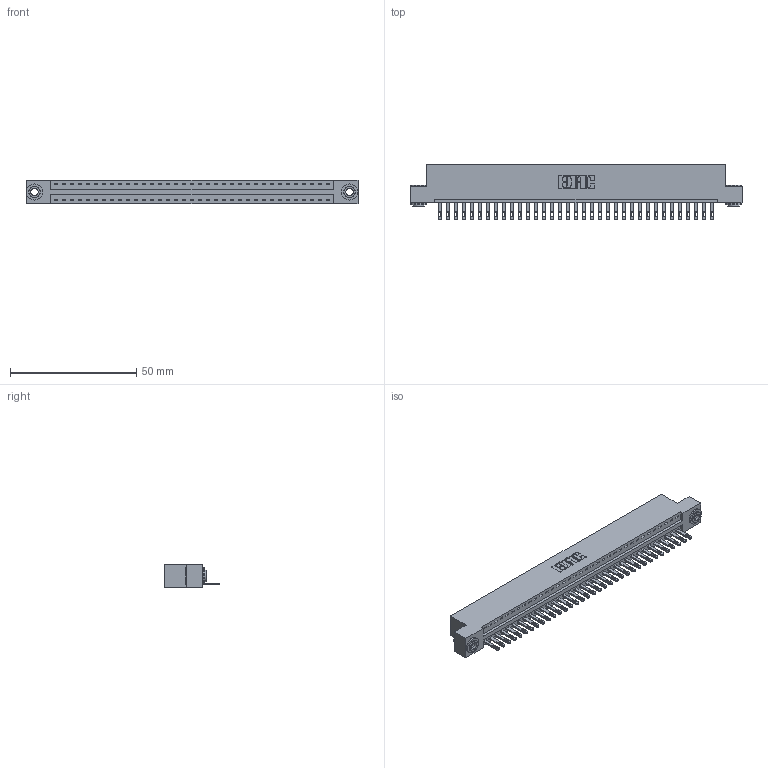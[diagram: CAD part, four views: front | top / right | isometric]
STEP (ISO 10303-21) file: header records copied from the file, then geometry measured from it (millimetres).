
FILE_DESCRIPTION (( 'STEP AP203' ), '1' );
FILE_NAME ('346-035-500-103.STEP', '2022-05-06T22:17:13', ( '' ), ( '' ), 'SwSTEP 2.0', 'SolidWorks 2020', '' );
FILE_SCHEMA (( 'CONFIG_CONTROL_DESIGN' ));
Length unit declared in the file: inch
Products named in the file (4): 345-250-002_345-250-002-102; 346 Part_Flush Mounting Lugs - 0.156 Dia-TH; 345-292-001_345-293-100; 346-035-500-103
Assembly tree (38 placements, depth 2):
  346-035-500-103
    346 Part_Flush Mounting Lugs - 0.156 Dia-TH
    345-292-001_345-293-100  x35
    345-250-002_345-250-002-102  x2
Bounding box: 131.7 x 21.84 x 9.4 mm (x, y, z)
Volume: 12581.2 mm3; surface area: 15982.4 mm2
Topology: 38 solids, 38 shells, 2064 faces, 6321 edges, 4210 vertices
Faces by surface type: plane 1290, cylinder 766, cone 8
Entity records: 23660 total; most frequent: CARTESIAN_POINT 4038, ORIENTED_EDGE 3998, DIRECTION 3603, EDGE_CURVE 1999, LINE 1699, VECTOR 1699, VERTEX_POINT 1330, AXIS2_PLACEMENT_3D 952
